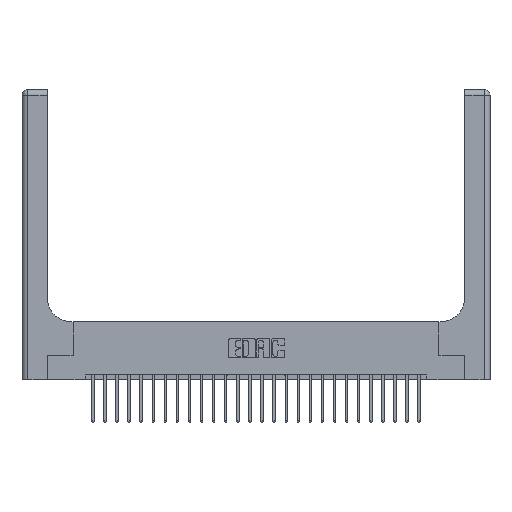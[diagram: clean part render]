
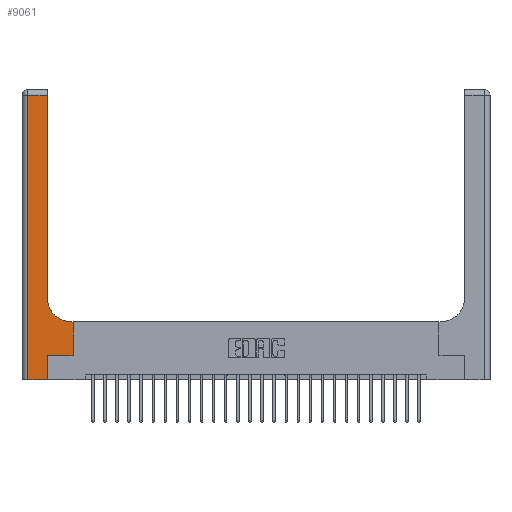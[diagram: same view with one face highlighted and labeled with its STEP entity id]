
A CAD part, top view. The second image highlights one B-rep face of the part: STEP entity #9061.
In plain terms, the highlighted planar face has unit normal (0, 0, 1).
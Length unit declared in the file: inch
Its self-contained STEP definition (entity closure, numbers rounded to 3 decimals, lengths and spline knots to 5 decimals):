
#206 = DIRECTION ( 'NONE',  ( -1., 0., 0. ) ) ;
#375 = CARTESIAN_POINT ( 'NONE',  ( 0.26, 2.94, 0.37 ) ) ;
#560 = VERTEX_POINT ( 'NONE', #6218 ) ;
#649 = DIRECTION ( 'NONE',  ( 1., 0., 0. ) ) ;
#841 = CARTESIAN_POINT ( 'NONE',  ( 0., 2.94, 0.37 ) ) ;
#2211 = VECTOR ( 'NONE', #7961, 39.37008 ) ;
#3014 = DIRECTION ( 'NONE',  ( 1., 0., 0. ) ) ;
#3418 = CARTESIAN_POINT ( 'NONE',  ( 0.528, 0.6, 0.37 ) ) ;
#3720 = CARTESIAN_POINT ( 'NONE',  ( 0.06, 3., 0.37 ) ) ;
#3814 = FACE_OUTER_BOUND ( 'NONE', #17712, .T. ) ;
#3970 = DIRECTION ( 'NONE',  ( 0., -1., 0. ) ) ;
#4358 = ORIENTED_EDGE ( 'NONE', *, *, #6109, .T. ) ;
#4387 = VERTEX_POINT ( 'NONE', #22971 ) ;
#4442 = EDGE_CURVE ( 'NONE', #8846, #4858, #15386, .T. ) ;
#4531 = CIRCLE ( 'NONE', #22077, 0.25 ) ;
#4532 = AXIS2_PLACEMENT_3D ( 'NONE', #10342, #19981, #18293 ) ;
#4858 = VERTEX_POINT ( 'NONE', #3418 ) ;
#5016 = ORIENTED_EDGE ( 'NONE', *, *, #21712, .T. ) ;
#5018 = VERTEX_POINT ( 'NONE', #375 ) ;
#5076 = VECTOR ( 'NONE', #3014, 39.37008 ) ;
#5439 = EDGE_CURVE ( 'NONE', #4858, #19524, #18254, .T. ) ;
#5650 = DIRECTION ( 'NONE',  ( 1., 0., 0. ) ) ;
#5990 = CARTESIAN_POINT ( 'NONE',  ( 0.26, 3., 0.37 ) ) ;
#6109 = EDGE_CURVE ( 'NONE', #19524, #560, #4531, .T. ) ;
#6218 = CARTESIAN_POINT ( 'NONE',  ( 0.26, 0.85, 0.37 ) ) ;
#6440 = VERTEX_POINT ( 'NONE', #16603 ) ;
#6720 = DIRECTION ( 'NONE',  ( 0., 1., 0. ) ) ;
#6822 = VECTOR ( 'NONE', #24743, 39.37008 ) ;
#7561 = VECTOR ( 'NONE', #649, 39.37008 ) ;
#7621 = VECTOR ( 'NONE', #3970, 39.37008 ) ;
#7847 = CARTESIAN_POINT ( 'NONE',  ( 0.26, 0.6, 0.37 ) ) ;
#7961 = DIRECTION ( 'NONE',  ( 0., 1., 0. ) ) ;
#8292 = CARTESIAN_POINT ( 'NONE',  ( 0.265, 0.25, 0.37 ) ) ;
#8667 = LINE ( 'NONE', #16621, #5076 ) ;
#8846 = VERTEX_POINT ( 'NONE', #18322 ) ;
#9061 = ADVANCED_FACE ( 'NONE', ( #3814 ), #15851, .F. ) ;
#9547 = VECTOR ( 'NONE', #11067, 39.37008 ) ;
#9961 = ORIENTED_EDGE ( 'NONE', *, *, #23208, .T. ) ;
#10342 = CARTESIAN_POINT ( 'NONE',  ( 0., 3., 0.37 ) ) ;
#10901 = CARTESIAN_POINT ( 'NONE',  ( 0.265, 0., 0.37 ) ) ;
#10958 = VERTEX_POINT ( 'NONE', #11601 ) ;
#11067 = DIRECTION ( 'NONE',  ( 0., 1., 0. ) ) ;
#11601 = CARTESIAN_POINT ( 'NONE',  ( 0.06, 0., 0.37 ) ) ;
#11996 = ORIENTED_EDGE ( 'NONE', *, *, #4442, .T. ) ;
#13316 = VECTOR ( 'NONE', #206, 39.37008 ) ;
#14615 = ORIENTED_EDGE ( 'NONE', *, *, #24494, .T. ) ;
#14876 = ORIENTED_EDGE ( 'NONE', *, *, #23715, .T. ) ;
#15386 = LINE ( 'NONE', #17208, #9547 ) ;
#15474 = DIRECTION ( 'NONE',  ( 0., 0., -1. ) ) ;
#15851 = PLANE ( 'NONE',  #4532 ) ;
#16603 = CARTESIAN_POINT ( 'NONE',  ( 0.06, 2.94, 0.37 ) ) ;
#16621 = CARTESIAN_POINT ( 'NONE',  ( 0., 0., 0.37 ) ) ;
#17173 = LINE ( 'NONE', #10901, #20910 ) ;
#17208 = CARTESIAN_POINT ( 'NONE',  ( 0.528, 0.25, 0.37 ) ) ;
#17230 = ORIENTED_EDGE ( 'NONE', *, *, #5439, .T. ) ;
#17712 = EDGE_LOOP ( 'NONE', ( #14615, #19505, #5016, #14876, #9961, #22630, #11996, #17230, #4358 ) ) ;
#17877 = LINE ( 'NONE', #5990, #2211 ) ;
#18107 = VERTEX_POINT ( 'NONE', #19527 ) ;
#18195 = LINE ( 'NONE', #8292, #7561 ) ;
#18254 = LINE ( 'NONE', #7847, #13316 ) ;
#18293 = DIRECTION ( 'NONE',  ( -1., 0., 0. ) ) ;
#18322 = CARTESIAN_POINT ( 'NONE',  ( 0.528, 0.25, 0.37 ) ) ;
#19505 = ORIENTED_EDGE ( 'NONE', *, *, #24581, .T. ) ;
#19524 = VERTEX_POINT ( 'NONE', #22664 ) ;
#19527 = CARTESIAN_POINT ( 'NONE',  ( 0.265, 0.25, 0.37 ) ) ;
#19981 = DIRECTION ( 'NONE',  ( 0., 0., -1. ) ) ;
#19995 = EDGE_CURVE ( 'NONE', #18107, #8846, #18195, .T. ) ;
#20910 = VECTOR ( 'NONE', #6720, 39.37008 ) ;
#21447 = CARTESIAN_POINT ( 'NONE',  ( 0.51, 0.85, 0.37 ) ) ;
#21712 = EDGE_CURVE ( 'NONE', #6440, #10958, #25777, .T. ) ;
#22077 = AXIS2_PLACEMENT_3D ( 'NONE', #21447, #15474, #5650 ) ;
#22412 = LINE ( 'NONE', #841, #6822 ) ;
#22630 = ORIENTED_EDGE ( 'NONE', *, *, #19995, .T. ) ;
#22664 = CARTESIAN_POINT ( 'NONE',  ( 0.51, 0.6, 0.37 ) ) ;
#22971 = CARTESIAN_POINT ( 'NONE',  ( 0.265, 0., 0.37 ) ) ;
#23208 = EDGE_CURVE ( 'NONE', #4387, #18107, #17173, .T. ) ;
#23715 = EDGE_CURVE ( 'NONE', #10958, #4387, #8667, .T. ) ;
#24494 = EDGE_CURVE ( 'NONE', #560, #5018, #17877, .T. ) ;
#24581 = EDGE_CURVE ( 'NONE', #5018, #6440, #22412, .T. ) ;
#24743 = DIRECTION ( 'NONE',  ( -1., 0., 0. ) ) ;
#25777 = LINE ( 'NONE', #3720, #7621 ) ;
